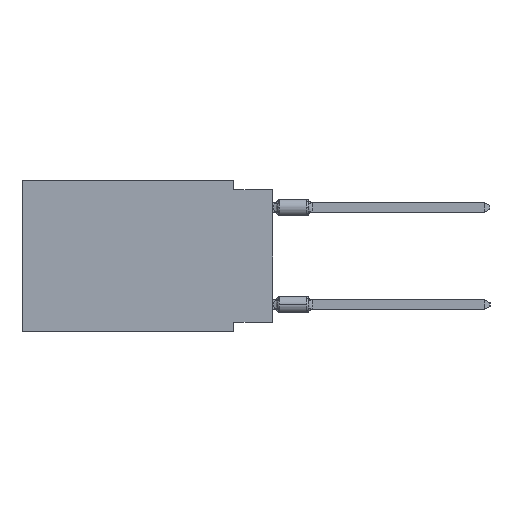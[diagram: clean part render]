
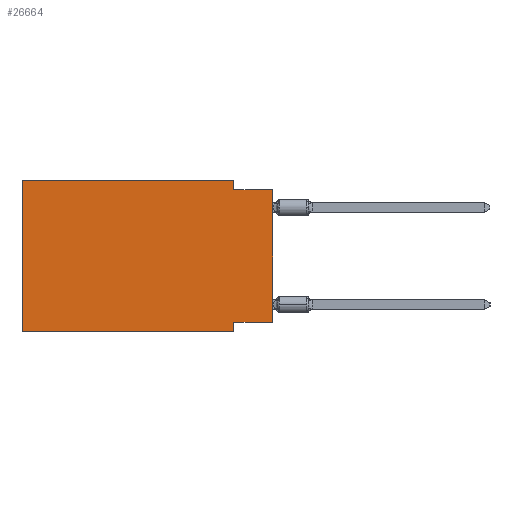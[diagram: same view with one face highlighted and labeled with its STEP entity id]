
A CAD part, left-side view. The second image highlights one B-rep face of the part: STEP entity #26664.
In plain terms, the highlighted planar face has unit normal (-1, 0, 0).
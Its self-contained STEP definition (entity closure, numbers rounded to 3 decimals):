
#570 = VERTEX_POINT ( 'NONE', #4304 ) ;
#684 = VERTEX_POINT ( 'NONE', #4987 ) ;
#845 = FACE_OUTER_BOUND ( 'NONE', #20051, .T. ) ;
#2033 = VERTEX_POINT ( 'NONE', #14121 ) ;
#2115 = VERTEX_POINT ( 'NONE', #16443 ) ;
#2290 = VECTOR ( 'NONE', #10801, 1000. ) ;
#2621 = DIRECTION ( 'NONE',  ( 0., 0., -1. ) ) ;
#2646 = VECTOR ( 'NONE', #21431, 1000. ) ;
#2691 = EDGE_CURVE ( 'NONE', #11390, #24270, #7099, .T. ) ;
#2758 = PLANE ( 'NONE',  #15523 ) ;
#2954 = VECTOR ( 'NONE', #21457, 1000. ) ;
#4304 = CARTESIAN_POINT ( 'NONE',  ( 0., 2.54, -9.906 ) ) ;
#4687 = DIRECTION ( 'NONE',  ( 1., 0., 0. ) ) ;
#4803 = EDGE_CURVE ( 'NONE', #2033, #2115, #25530, .T. ) ;
#4817 = CARTESIAN_POINT ( 'NONE',  ( 0., 0., 0. ) ) ;
#4883 = ORIENTED_EDGE ( 'NONE', *, *, #2691, .F. ) ;
#4987 = CARTESIAN_POINT ( 'NONE',  ( 0., 0., -0.635 ) ) ;
#5820 = DIRECTION ( 'NONE',  ( 0., -1., 0. ) ) ;
#5961 = LINE ( 'NONE', #8145, #20283 ) ;
#6951 = CARTESIAN_POINT ( 'NONE',  ( 0., 0., -0.635 ) ) ;
#7099 = LINE ( 'NONE', #25250, #20264 ) ;
#7197 = ORIENTED_EDGE ( 'NONE', *, *, #17311, .T. ) ;
#8145 = CARTESIAN_POINT ( 'NONE',  ( 0., 16.383, 0. ) ) ;
#8774 = EDGE_CURVE ( 'NONE', #24270, #684, #13242, .T. ) ;
#9175 = CARTESIAN_POINT ( 'NONE',  ( 0., 2.54, -0.635 ) ) ;
#10486 = EDGE_CURVE ( 'NONE', #2115, #11390, #5961, .T. ) ;
#10801 = DIRECTION ( 'NONE',  ( 0., 0., -1. ) ) ;
#11390 = VERTEX_POINT ( 'NONE', #12703 ) ;
#12703 = CARTESIAN_POINT ( 'NONE',  ( 0., 2.54, 0. ) ) ;
#13242 = LINE ( 'NONE', #6951, #18097 ) ;
#13937 = DIRECTION ( 'NONE',  ( 0., 1., 0. ) ) ;
#14099 = VERTEX_POINT ( 'NONE', #15937 ) ;
#14121 = CARTESIAN_POINT ( 'NONE',  ( 0., 16.383, -9.906 ) ) ;
#14764 = CARTESIAN_POINT ( 'NONE',  ( 0., 2.54, -9.906 ) ) ;
#15523 = AXIS2_PLACEMENT_3D ( 'NONE', #25686, #4687, #2621 ) ;
#15670 = ORIENTED_EDGE ( 'NONE', *, *, #18985, .F. ) ;
#15937 = CARTESIAN_POINT ( 'NONE',  ( 0., 2.54, -9.271 ) ) ;
#16443 = CARTESIAN_POINT ( 'NONE',  ( 0., 16.383, 0. ) ) ;
#16567 = LINE ( 'NONE', #4817, #2954 ) ;
#17215 = LINE ( 'NONE', #14764, #2290 ) ;
#17311 = EDGE_CURVE ( 'NONE', #26600, #684, #16567, .T. ) ;
#17484 = CARTESIAN_POINT ( 'NONE',  ( 0., 16.383, 0. ) ) ;
#18097 = VECTOR ( 'NONE', #26169, 1000. ) ;
#18186 = LINE ( 'NONE', #21987, #22206 ) ;
#18985 = EDGE_CURVE ( 'NONE', #14099, #570, #17215, .T. ) ;
#19886 = CARTESIAN_POINT ( 'NONE',  ( 0., 16.383, -9.906 ) ) ;
#20051 = EDGE_LOOP ( 'NONE', ( #7197, #25905, #4883, #21015, #20656, #26202, #15670, #26307 ) ) ;
#20264 = VECTOR ( 'NONE', #25386, 1000. ) ;
#20283 = VECTOR ( 'NONE', #5820, 1000. ) ;
#20656 = ORIENTED_EDGE ( 'NONE', *, *, #4803, .F. ) ;
#21015 = ORIENTED_EDGE ( 'NONE', *, *, #10486, .F. ) ;
#21431 = DIRECTION ( 'NONE',  ( 0., 0., 1. ) ) ;
#21457 = DIRECTION ( 'NONE',  ( 0., 0., 1. ) ) ;
#21987 = CARTESIAN_POINT ( 'NONE',  ( 0., 0., -9.271 ) ) ;
#22206 = VECTOR ( 'NONE', #13937, 1000. ) ;
#23562 = DIRECTION ( 'NONE',  ( 0., -1., 0. ) ) ;
#24270 = VERTEX_POINT ( 'NONE', #9175 ) ;
#24361 = EDGE_CURVE ( 'NONE', #26600, #14099, #18186, .T. ) ;
#24614 = EDGE_CURVE ( 'NONE', #2033, #570, #25733, .T. ) ;
#24646 = VECTOR ( 'NONE', #23562, 1000. ) ;
#25250 = CARTESIAN_POINT ( 'NONE',  ( 0., 2.54, 0. ) ) ;
#25386 = DIRECTION ( 'NONE',  ( 0., 0., -1. ) ) ;
#25530 = LINE ( 'NONE', #17484, #2646 ) ;
#25686 = CARTESIAN_POINT ( 'NONE',  ( 0., 16.383, 0. ) ) ;
#25733 = LINE ( 'NONE', #19886, #24646 ) ;
#25821 = CARTESIAN_POINT ( 'NONE',  ( 0., 0., -9.271 ) ) ;
#25905 = ORIENTED_EDGE ( 'NONE', *, *, #8774, .F. ) ;
#26169 = DIRECTION ( 'NONE',  ( 0., -1., 0. ) ) ;
#26202 = ORIENTED_EDGE ( 'NONE', *, *, #24614, .T. ) ;
#26307 = ORIENTED_EDGE ( 'NONE', *, *, #24361, .F. ) ;
#26600 = VERTEX_POINT ( 'NONE', #25821 ) ;
#26664 = ADVANCED_FACE ( 'NONE', ( #845 ), #2758, .F. ) ;
